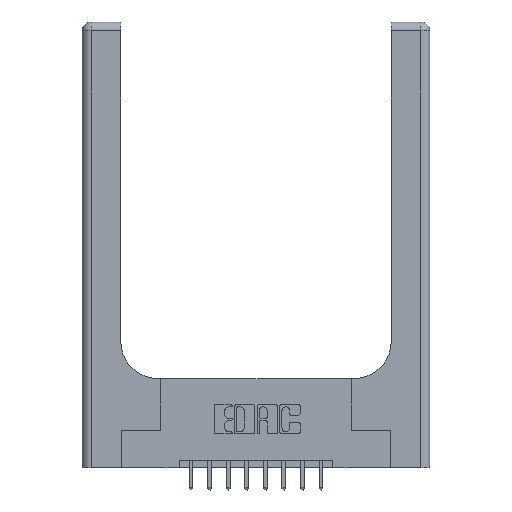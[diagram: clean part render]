
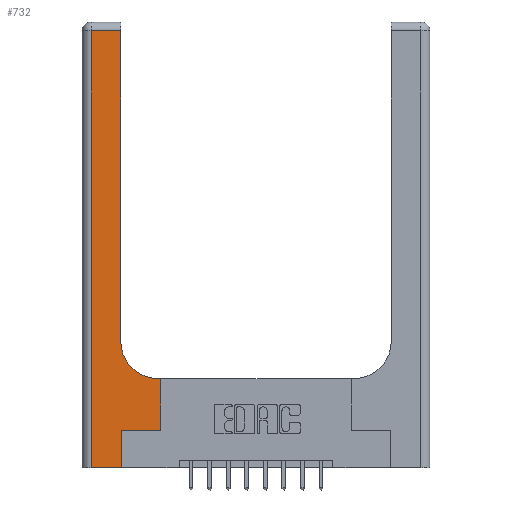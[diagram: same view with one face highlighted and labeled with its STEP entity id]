
A CAD part, top view. The second image highlights one B-rep face of the part: STEP entity #732.
In plain terms, the highlighted planar face has unit normal (0, 0, 1).
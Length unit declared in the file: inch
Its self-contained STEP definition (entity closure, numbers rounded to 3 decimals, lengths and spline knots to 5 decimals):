
#125 = CARTESIAN_POINT ( 'NONE',  ( 0.265, 0., 0.37 ) ) ;
#231 = VERTEX_POINT ( 'NONE', #5861 ) ;
#525 = DIRECTION ( 'NONE',  ( 1., 0., 0. ) ) ;
#628 = AXIS2_PLACEMENT_3D ( 'NONE', #5502, #11237, #9990 ) ;
#655 = EDGE_CURVE ( 'NONE', #5787, #9585, #9123, .T. ) ;
#732 = ADVANCED_FACE ( 'NONE', ( #11596 ), #10429, .F. ) ;
#913 = LINE ( 'NONE', #8128, #8535 ) ;
#989 = CARTESIAN_POINT ( 'NONE',  ( 0.51, 0.6, 0.37 ) ) ;
#1077 = EDGE_CURVE ( 'NONE', #8954, #7995, #3664, .T. ) ;
#1635 = DIRECTION ( 'NONE',  ( 0., 1., 0. ) ) ;
#1675 = CARTESIAN_POINT ( 'NONE',  ( 0.528, 0.6, 0.37 ) ) ;
#2001 = CARTESIAN_POINT ( 'NONE',  ( 0.265, 0., 0.37 ) ) ;
#2045 = LINE ( 'NONE', #11800, #9937 ) ;
#2159 = LINE ( 'NONE', #2001, #11546 ) ;
#2346 = ORIENTED_EDGE ( 'NONE', *, *, #11490, .T. ) ;
#2502 = ORIENTED_EDGE ( 'NONE', *, *, #5392, .T. ) ;
#2734 = EDGE_CURVE ( 'NONE', #11505, #11519, #9372, .T. ) ;
#3405 = VECTOR ( 'NONE', #10619, 39.37008 ) ;
#3556 = CARTESIAN_POINT ( 'NONE',  ( 0., 3., 0.37 ) ) ;
#3664 = LINE ( 'NONE', #4500, #14242 ) ;
#3737 = EDGE_LOOP ( 'NONE', ( #11662, #3778, #2502, #2346, #4846, #3905, #5727, #9386, #15039 ) ) ;
#3778 = ORIENTED_EDGE ( 'NONE', *, *, #1077, .T. ) ;
#3849 = VECTOR ( 'NONE', #3927, 39.37008 ) ;
#3905 = ORIENTED_EDGE ( 'NONE', *, *, #655, .T. ) ;
#3927 = DIRECTION ( 'NONE',  ( 0., 1., 0. ) ) ;
#4500 = CARTESIAN_POINT ( 'NONE',  ( 0., 2.94, 0.37 ) ) ;
#4507 = EDGE_CURVE ( 'NONE', #13858, #5787, #2159, .T. ) ;
#4589 = EDGE_CURVE ( 'NONE', #9861, #11505, #5964, .T. ) ;
#4846 = ORIENTED_EDGE ( 'NONE', *, *, #4507, .T. ) ;
#4855 = CARTESIAN_POINT ( 'NONE',  ( 0.06, 2.94, 0.37 ) ) ;
#5392 = EDGE_CURVE ( 'NONE', #7995, #231, #2045, .T. ) ;
#5502 = CARTESIAN_POINT ( 'NONE',  ( 0.51, 0.85, 0.37 ) ) ;
#5624 = DIRECTION ( 'NONE',  ( 1., 0., 0. ) ) ;
#5727 = ORIENTED_EDGE ( 'NONE', *, *, #14296, .T. ) ;
#5787 = VERTEX_POINT ( 'NONE', #8519 ) ;
#5861 = CARTESIAN_POINT ( 'NONE',  ( 0.06, 0., 0.37 ) ) ;
#5887 = CARTESIAN_POINT ( 'NONE',  ( 0.26, 0.6, 0.37 ) ) ;
#5964 = LINE ( 'NONE', #5887, #3405 ) ;
#6770 = DIRECTION ( 'NONE',  ( 0., 1., 0. ) ) ;
#7039 = DIRECTION ( 'NONE',  ( 0., 0., -1. ) ) ;
#7326 = CARTESIAN_POINT ( 'NONE',  ( 0.528, 0.25, 0.37 ) ) ;
#7765 = CARTESIAN_POINT ( 'NONE',  ( 0.528, 0.25, 0.37 ) ) ;
#7856 = AXIS2_PLACEMENT_3D ( 'NONE', #3556, #7039, #10664 ) ;
#7995 = VERTEX_POINT ( 'NONE', #4855 ) ;
#8007 = CARTESIAN_POINT ( 'NONE',  ( 0.26, 2.94, 0.37 ) ) ;
#8128 = CARTESIAN_POINT ( 'NONE',  ( 0., 0., 0.37 ) ) ;
#8519 = CARTESIAN_POINT ( 'NONE',  ( 0.265, 0.25, 0.37 ) ) ;
#8535 = VECTOR ( 'NONE', #5624, 39.37008 ) ;
#8633 = LINE ( 'NONE', #7326, #8811 ) ;
#8720 = CARTESIAN_POINT ( 'NONE',  ( 0.26, 3., 0.37 ) ) ;
#8811 = VECTOR ( 'NONE', #1635, 39.37008 ) ;
#8954 = VERTEX_POINT ( 'NONE', #8007 ) ;
#9123 = LINE ( 'NONE', #11205, #13819 ) ;
#9372 = CIRCLE ( 'NONE', #628, 0.25 ) ;
#9386 = ORIENTED_EDGE ( 'NONE', *, *, #4589, .T. ) ;
#9585 = VERTEX_POINT ( 'NONE', #7765 ) ;
#9861 = VERTEX_POINT ( 'NONE', #1675 ) ;
#9937 = VECTOR ( 'NONE', #14241, 39.37008 ) ;
#9990 = DIRECTION ( 'NONE',  ( 1., 0., 0. ) ) ;
#10300 = EDGE_CURVE ( 'NONE', #11519, #8954, #14825, .T. ) ;
#10429 = PLANE ( 'NONE',  #7856 ) ;
#10619 = DIRECTION ( 'NONE',  ( -1., 0., 0. ) ) ;
#10664 = DIRECTION ( 'NONE',  ( -1., 0., 0. ) ) ;
#11205 = CARTESIAN_POINT ( 'NONE',  ( 0.265, 0.25, 0.37 ) ) ;
#11237 = DIRECTION ( 'NONE',  ( 0., 0., -1. ) ) ;
#11490 = EDGE_CURVE ( 'NONE', #231, #13858, #913, .T. ) ;
#11505 = VERTEX_POINT ( 'NONE', #989 ) ;
#11519 = VERTEX_POINT ( 'NONE', #14113 ) ;
#11546 = VECTOR ( 'NONE', #6770, 39.37008 ) ;
#11596 = FACE_OUTER_BOUND ( 'NONE', #3737, .T. ) ;
#11662 = ORIENTED_EDGE ( 'NONE', *, *, #10300, .T. ) ;
#11800 = CARTESIAN_POINT ( 'NONE',  ( 0.06, 3., 0.37 ) ) ;
#13819 = VECTOR ( 'NONE', #525, 39.37008 ) ;
#13858 = VERTEX_POINT ( 'NONE', #125 ) ;
#14113 = CARTESIAN_POINT ( 'NONE',  ( 0.26, 0.85, 0.37 ) ) ;
#14155 = DIRECTION ( 'NONE',  ( -1., 0., 0. ) ) ;
#14241 = DIRECTION ( 'NONE',  ( 0., -1., 0. ) ) ;
#14242 = VECTOR ( 'NONE', #14155, 39.37008 ) ;
#14296 = EDGE_CURVE ( 'NONE', #9585, #9861, #8633, .T. ) ;
#14825 = LINE ( 'NONE', #8720, #3849 ) ;
#15039 = ORIENTED_EDGE ( 'NONE', *, *, #2734, .T. ) ;
